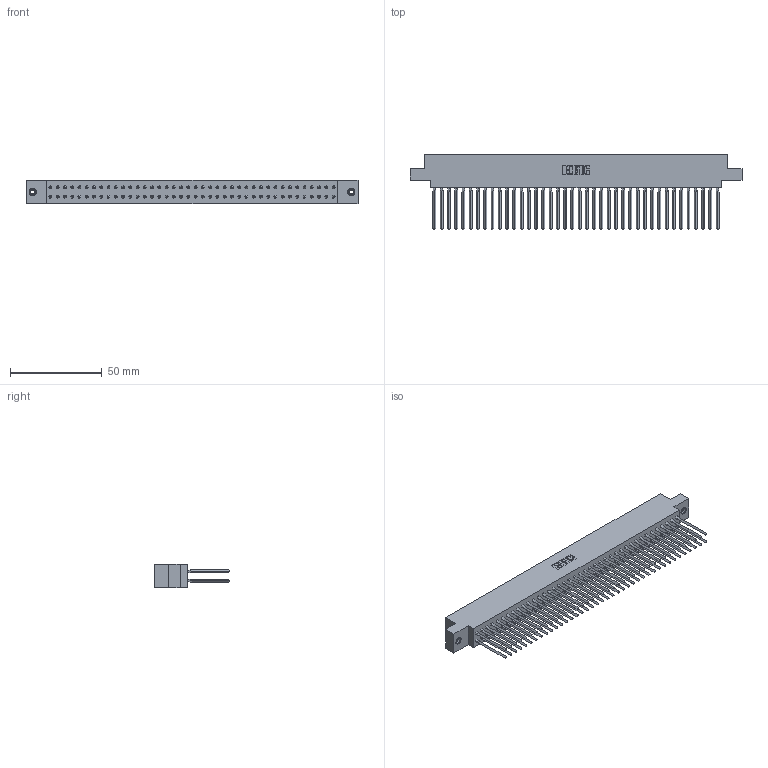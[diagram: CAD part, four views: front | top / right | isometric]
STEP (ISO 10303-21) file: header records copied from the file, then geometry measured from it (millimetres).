
FILE_DESCRIPTION (( 'STEP AP203' ), '1' );
FILE_NAME ('317-080-543-808.STEP', '2020-02-28T09:28:03', ( '' ), ( '' ), 'SwSTEP 2.0', 'SolidWorks 2016', '' );
FILE_SCHEMA (( 'CONFIG_CONTROL_DESIGN' ));
Length unit declared in the file: inch
Products named in the file (4): 317-290-001_543; 345-250-001_345-250-003-102; 317-080-543-808; 317 Part_.156 Dia - TI
Assembly tree (83 placements, depth 2):
  317-080-543-808
    317 Part_.156 Dia - TI
    317-290-001_543  x80
    345-250-001_345-250-003-102  x2
Bounding box: 181.2 x 41.15 x 12.7 mm (x, y, z)
Volume: 30735.6 mm3; surface area: 46570.7 mm2
Topology: 83 solids, 83 shells, 7282 faces, 20171 edges, 12986 vertices
Faces by surface type: plane 5930, cylinder 1016, bspline 320, cone 12, torus 4
Entity records: 59285 total; most frequent: CARTESIAN_POINT 10730, ORIENTED_EDGE 10222, DIRECTION 8567, EDGE_CURVE 5111, LINE 4835, VECTOR 4835, VERTEX_POINT 3397, AXIS2_PLACEMENT_3D 1866
